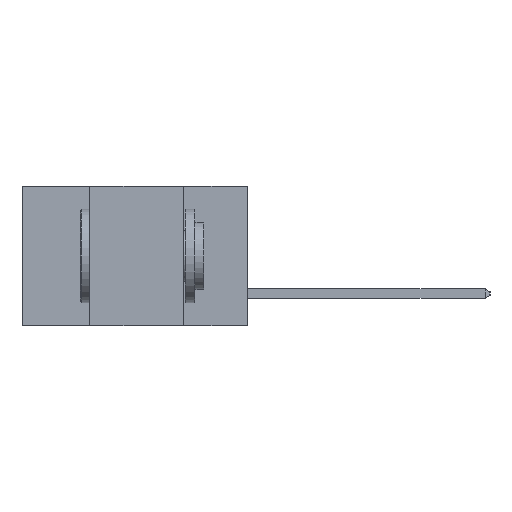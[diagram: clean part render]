
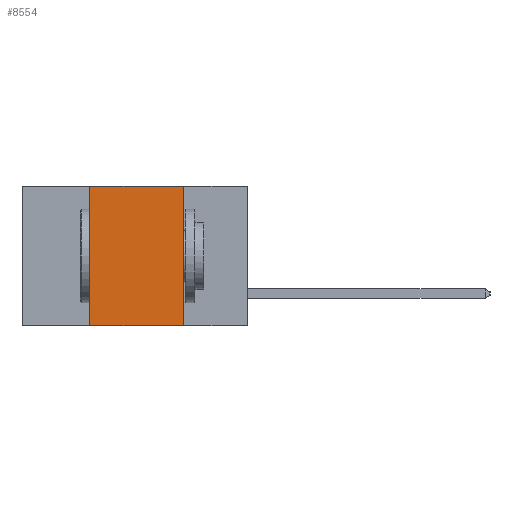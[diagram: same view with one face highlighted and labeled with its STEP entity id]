
A CAD part, left-side view. The second image highlights one B-rep face of the part: STEP entity #8554.
In plain terms, the highlighted planar face has unit normal (-1, 0, 0).
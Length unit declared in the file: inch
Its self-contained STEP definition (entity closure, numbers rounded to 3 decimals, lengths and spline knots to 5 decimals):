
#360 = EDGE_LOOP ( 'NONE', ( #9246, #9273, #9320, #9382 ) ) ;
#769 = VERTEX_POINT ( 'NONE', #5496 ) ;
#1237 = VERTEX_POINT ( 'NONE', #1453 ) ;
#1453 = CARTESIAN_POINT ( 'NONE',  ( 0., 0.17, 0. ) ) ;
#2299 = CARTESIAN_POINT ( 'NONE',  ( 0., 0.6, 0. ) ) ;
#2617 = VERTEX_POINT ( 'NONE', #8644 ) ;
#3391 = LINE ( 'NONE', #10054, #5800 ) ;
#3651 = EDGE_CURVE ( 'NONE', #4941, #769, #12558, .T. ) ;
#4343 = EDGE_CURVE ( 'NONE', #4941, #2617, #11618, .T. ) ;
#4357 = DIRECTION ( 'NONE',  ( 1., 0., 0. ) ) ;
#4941 = VERTEX_POINT ( 'NONE', #6221 ) ;
#5029 = EDGE_CURVE ( 'NONE', #2617, #1237, #10824, .T. ) ;
#5496 = CARTESIAN_POINT ( 'NONE',  ( 0., 0.17, -0.37 ) ) ;
#5513 = VECTOR ( 'NONE', #5756, 39.37008 ) ;
#5756 = DIRECTION ( 'NONE',  ( 0., -1., 0. ) ) ;
#5787 = CARTESIAN_POINT ( 'NONE',  ( 0., 0.6, 0. ) ) ;
#5800 = VECTOR ( 'NONE', #11030, 39.37008 ) ;
#6011 = VECTOR ( 'NONE', #8359, 39.37008 ) ;
#6221 = CARTESIAN_POINT ( 'NONE',  ( 0., 0.42, -0.37 ) ) ;
#6395 = EDGE_CURVE ( 'NONE', #1237, #769, #3391, .T. ) ;
#7177 = FACE_OUTER_BOUND ( 'NONE', #360, .T. ) ;
#8359 = DIRECTION ( 'NONE',  ( 0., 0., 1. ) ) ;
#8434 = CARTESIAN_POINT ( 'NONE',  ( 0., 0.42, -0.37 ) ) ;
#8554 = ADVANCED_FACE ( 'NONE', ( #7177 ), #10394, .F. ) ;
#8644 = CARTESIAN_POINT ( 'NONE',  ( 0., 0.42, 0. ) ) ;
#9246 = ORIENTED_EDGE ( 'NONE', *, *, #6395, .F. ) ;
#9273 = ORIENTED_EDGE ( 'NONE', *, *, #5029, .F. ) ;
#9320 = ORIENTED_EDGE ( 'NONE', *, *, #4343, .F. ) ;
#9382 = ORIENTED_EDGE ( 'NONE', *, *, #3651, .T. ) ;
#9664 = VECTOR ( 'NONE', #11028, 39.37008 ) ;
#10054 = CARTESIAN_POINT ( 'NONE',  ( 0., 0.17, -0.37 ) ) ;
#10394 = PLANE ( 'NONE',  #12957 ) ;
#10824 = LINE ( 'NONE', #5787, #5513 ) ;
#11028 = DIRECTION ( 'NONE',  ( 0., -1., 0. ) ) ;
#11030 = DIRECTION ( 'NONE',  ( 0., 0., -1. ) ) ;
#11375 = DIRECTION ( 'NONE',  ( 0., 0., -1. ) ) ;
#11618 = LINE ( 'NONE', #8434, #6011 ) ;
#12167 = CARTESIAN_POINT ( 'NONE',  ( 0., 0.6, -0.37 ) ) ;
#12558 = LINE ( 'NONE', #12167, #9664 ) ;
#12957 = AXIS2_PLACEMENT_3D ( 'NONE', #2299, #4357, #11375 ) ;
